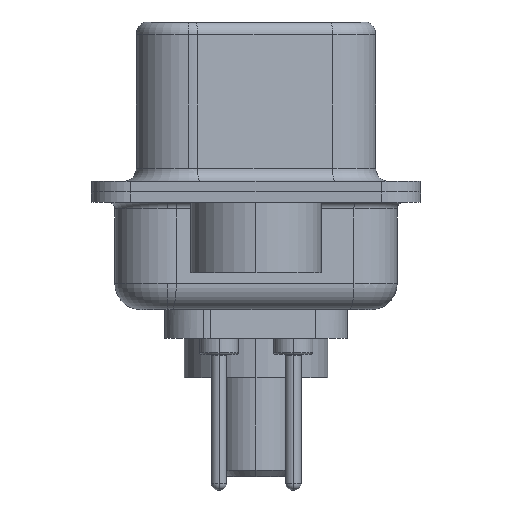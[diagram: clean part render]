
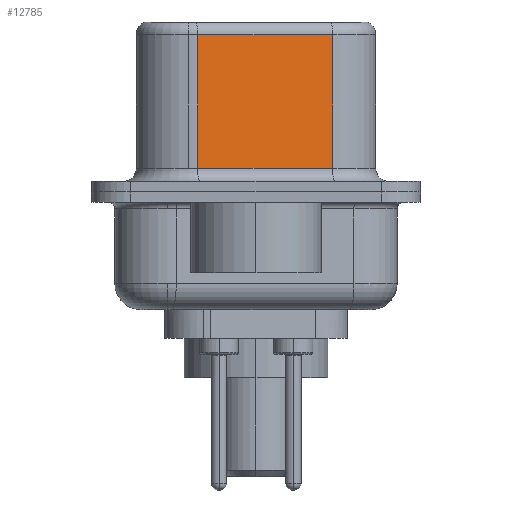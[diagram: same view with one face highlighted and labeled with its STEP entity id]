
A CAD part, left-side view. The second image highlights one B-rep face of the part: STEP entity #12785.
In plain terms, the highlighted planar face has unit normal (-0.985, -0.174, 0).
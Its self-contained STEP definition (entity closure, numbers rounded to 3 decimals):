
#8 = DIRECTION ( 'NONE',  ( -0.174, 0.985, 0. ) ) ;
#119 = CARTESIAN_POINT ( 'NONE',  ( 4.58, -2.927, 6.02 ) ) ;
#168 = CARTESIAN_POINT ( 'NONE',  ( 3.67, 2.233, 6.52 ) ) ;
#924 = ORIENTED_EDGE ( 'NONE', *, *, #7668, .T. ) ;
#952 = ORIENTED_EDGE ( 'NONE', *, *, #5491, .T. ) ;
#1753 = DIRECTION ( 'NONE',  ( 0.174, -0.985, 0. ) ) ;
#2903 = CARTESIAN_POINT ( 'NONE',  ( 4.58, -2.927, 0.9 ) ) ;
#4142 = DIRECTION ( 'NONE',  ( 0., 0., -1. ) ) ;
#4319 = VECTOR ( 'NONE', #4142, 1000. ) ;
#4433 = VERTEX_POINT ( 'NONE', #119 ) ;
#4457 = VERTEX_POINT ( 'NONE', #13524 ) ;
#5491 = EDGE_CURVE ( 'NONE', #11885, #4457, #12874, .T. ) ;
#6167 = VERTEX_POINT ( 'NONE', #9558 ) ;
#6333 = VECTOR ( 'NONE', #8394, 1000. ) ;
#6460 = DIRECTION ( 'NONE',  ( 0.985, 0.174, 0. ) ) ;
#6664 = LINE ( 'NONE', #2903, #12192 ) ;
#6750 = FACE_OUTER_BOUND ( 'NONE', #12857, .T. ) ;
#7043 = VECTOR ( 'NONE', #7561, 1000. ) ;
#7124 = EDGE_CURVE ( 'NONE', #4433, #11885, #8969, .T. ) ;
#7561 = DIRECTION ( 'NONE',  ( 0., 0., -1. ) ) ;
#7668 = EDGE_CURVE ( 'NONE', #4457, #6167, #6664, .T. ) ;
#7883 = EDGE_CURVE ( 'NONE', #4433, #6167, #10189, .T. ) ;
#8255 = CARTESIAN_POINT ( 'NONE',  ( 4.58, -2.927, 6.02 ) ) ;
#8394 = DIRECTION ( 'NONE',  ( -0.174, 0.985, 0. ) ) ;
#8969 = LINE ( 'NONE', #8255, #6333 ) ;
#9316 = CARTESIAN_POINT ( 'NONE',  ( 3.67, 2.233, 6.02 ) ) ;
#9558 = CARTESIAN_POINT ( 'NONE',  ( 4.58, -2.927, 0.9 ) ) ;
#9774 = CARTESIAN_POINT ( 'NONE',  ( 4.58, -2.927, 6.52 ) ) ;
#10055 = CARTESIAN_POINT ( 'NONE',  ( 4.58, -2.927, 6.52 ) ) ;
#10189 = LINE ( 'NONE', #10055, #4319 ) ;
#10917 = PLANE ( 'NONE',  #12647 ) ;
#11097 = ORIENTED_EDGE ( 'NONE', *, *, #7124, .T. ) ;
#11885 = VERTEX_POINT ( 'NONE', #9316 ) ;
#12068 = ORIENTED_EDGE ( 'NONE', *, *, #7883, .F. ) ;
#12192 = VECTOR ( 'NONE', #1753, 1000. ) ;
#12647 = AXIS2_PLACEMENT_3D ( 'NONE', #9774, #6460, #8 ) ;
#12785 = ADVANCED_FACE ( 'NONE', ( #6750 ), #10917, .F. ) ;
#12857 = EDGE_LOOP ( 'NONE', ( #12068, #11097, #952, #924 ) ) ;
#12874 = LINE ( 'NONE', #168, #7043 ) ;
#13524 = CARTESIAN_POINT ( 'NONE',  ( 3.67, 2.233, 0.9 ) ) ;
